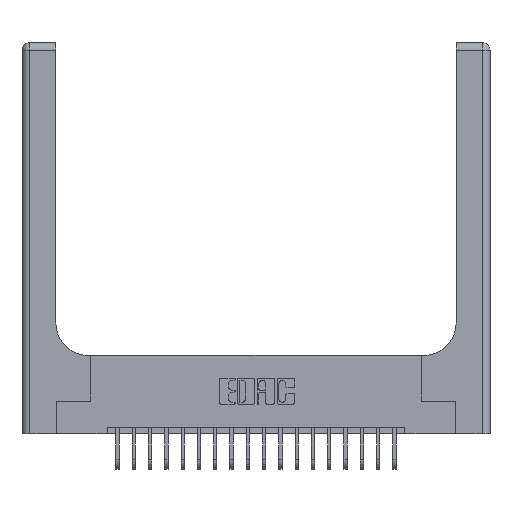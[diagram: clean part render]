
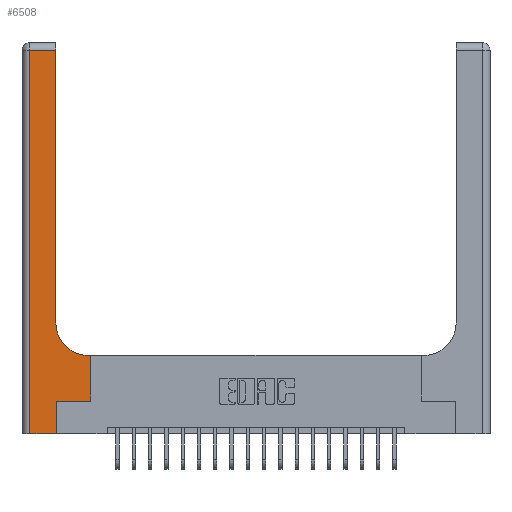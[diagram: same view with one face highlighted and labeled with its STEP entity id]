
A CAD part, top view. The second image highlights one B-rep face of the part: STEP entity #6508.
In plain terms, the highlighted planar face has unit normal (0, 0, 1).
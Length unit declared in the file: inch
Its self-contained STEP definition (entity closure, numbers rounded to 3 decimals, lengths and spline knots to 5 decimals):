
#472 = EDGE_CURVE ( 'NONE', #2801, #19625, #3547, .T. ) ;
#615 = CARTESIAN_POINT ( 'NONE',  ( 0.265, 0., 0.37 ) ) ;
#683 = PLANE ( 'NONE',  #11475 ) ;
#1580 = DIRECTION ( 'NONE',  ( 1., 0., 0. ) ) ;
#1695 = DIRECTION ( 'NONE',  ( 0., -1., 0. ) ) ;
#1717 = EDGE_CURVE ( 'NONE', #19625, #13800, #10769, .T. ) ;
#1804 = VECTOR ( 'NONE', #12880, 39.37008 ) ;
#1889 = CARTESIAN_POINT ( 'NONE',  ( 0.528, 0.25, 0.37 ) ) ;
#2115 = FACE_OUTER_BOUND ( 'NONE', #16311, .T. ) ;
#2153 = EDGE_CURVE ( 'NONE', #5515, #14715, #13797, .T. ) ;
#2319 = EDGE_CURVE ( 'NONE', #13633, #2801, #19051, .T. ) ;
#2414 = ORIENTED_EDGE ( 'NONE', *, *, #12610, .T. ) ;
#2652 = CARTESIAN_POINT ( 'NONE',  ( 0.51, 0.6, 0.37 ) ) ;
#2801 = VERTEX_POINT ( 'NONE', #17411 ) ;
#3007 = VERTEX_POINT ( 'NONE', #2652 ) ;
#3537 = EDGE_CURVE ( 'NONE', #10166, #3007, #11063, .T. ) ;
#3547 = LINE ( 'NONE', #15643, #15716 ) ;
#3594 = EDGE_CURVE ( 'NONE', #14715, #10166, #6774, .T. ) ;
#3761 = VECTOR ( 'NONE', #5128, 39.37008 ) ;
#4103 = VECTOR ( 'NONE', #11408, 39.37008 ) ;
#4941 = ORIENTED_EDGE ( 'NONE', *, *, #2153, .T. ) ;
#5128 = DIRECTION ( 'NONE',  ( -1., 0., 0. ) ) ;
#5199 = CIRCLE ( 'NONE', #8436, 0.25 ) ;
#5515 = VERTEX_POINT ( 'NONE', #12678 ) ;
#6261 = VECTOR ( 'NONE', #7864, 39.37008 ) ;
#6306 = DIRECTION ( 'NONE',  ( 1., 0., 0. ) ) ;
#6508 = ADVANCED_FACE ( 'NONE', ( #2115 ), #683, .F. ) ;
#6555 = VERTEX_POINT ( 'NONE', #8511 ) ;
#6585 = CARTESIAN_POINT ( 'NONE',  ( 0.528, 0.25, 0.37 ) ) ;
#6631 = LINE ( 'NONE', #12851, #6261 ) ;
#6774 = LINE ( 'NONE', #1889, #15116 ) ;
#7864 = DIRECTION ( 'NONE',  ( 0., 1., 0. ) ) ;
#8000 = CARTESIAN_POINT ( 'NONE',  ( 0.06, 0., 0.37 ) ) ;
#8436 = AXIS2_PLACEMENT_3D ( 'NONE', #11306, #12644, #6306 ) ;
#8511 = CARTESIAN_POINT ( 'NONE',  ( 0.26, 0.85, 0.37 ) ) ;
#9161 = EDGE_CURVE ( 'NONE', #13800, #5515, #18616, .T. ) ;
#9781 = ORIENTED_EDGE ( 'NONE', *, *, #472, .T. ) ;
#10166 = VERTEX_POINT ( 'NONE', #10931 ) ;
#10769 = LINE ( 'NONE', #16954, #17042 ) ;
#10931 = CARTESIAN_POINT ( 'NONE',  ( 0.528, 0.6, 0.37 ) ) ;
#11063 = LINE ( 'NONE', #18856, #1804 ) ;
#11306 = CARTESIAN_POINT ( 'NONE',  ( 0.51, 0.85, 0.37 ) ) ;
#11408 = DIRECTION ( 'NONE',  ( 0., 1., 0. ) ) ;
#11475 = AXIS2_PLACEMENT_3D ( 'NONE', #17960, #13020, #16248 ) ;
#11671 = CARTESIAN_POINT ( 'NONE',  ( 0.26, 2.94, 0.37 ) ) ;
#12589 = CARTESIAN_POINT ( 'NONE',  ( 0., 2.94, 0.37 ) ) ;
#12610 = EDGE_CURVE ( 'NONE', #6555, #13633, #6631, .T. ) ;
#12644 = DIRECTION ( 'NONE',  ( 0., 0., -1. ) ) ;
#12678 = CARTESIAN_POINT ( 'NONE',  ( 0.265, 0.25, 0.37 ) ) ;
#12851 = CARTESIAN_POINT ( 'NONE',  ( 0.26, 3., 0.37 ) ) ;
#12880 = DIRECTION ( 'NONE',  ( -1., 0., 0. ) ) ;
#12958 = EDGE_CURVE ( 'NONE', #3007, #6555, #5199, .T. ) ;
#13020 = DIRECTION ( 'NONE',  ( 0., 0., -1. ) ) ;
#13633 = VERTEX_POINT ( 'NONE', #11671 ) ;
#13797 = LINE ( 'NONE', #19872, #16083 ) ;
#13800 = VERTEX_POINT ( 'NONE', #19874 ) ;
#14033 = DIRECTION ( 'NONE',  ( 1., 0., 0. ) ) ;
#14189 = ORIENTED_EDGE ( 'NONE', *, *, #9161, .T. ) ;
#14715 = VERTEX_POINT ( 'NONE', #6585 ) ;
#15004 = ORIENTED_EDGE ( 'NONE', *, *, #3594, .T. ) ;
#15116 = VECTOR ( 'NONE', #19057, 39.37008 ) ;
#15643 = CARTESIAN_POINT ( 'NONE',  ( 0.06, 3., 0.37 ) ) ;
#15716 = VECTOR ( 'NONE', #1695, 39.37008 ) ;
#16083 = VECTOR ( 'NONE', #1580, 39.37008 ) ;
#16180 = ORIENTED_EDGE ( 'NONE', *, *, #3537, .T. ) ;
#16248 = DIRECTION ( 'NONE',  ( -1., 0., 0. ) ) ;
#16311 = EDGE_LOOP ( 'NONE', ( #2414, #17262, #9781, #16590, #14189, #4941, #15004, #16180, #17582 ) ) ;
#16590 = ORIENTED_EDGE ( 'NONE', *, *, #1717, .T. ) ;
#16954 = CARTESIAN_POINT ( 'NONE',  ( 0., 0., 0.37 ) ) ;
#17042 = VECTOR ( 'NONE', #14033, 39.37008 ) ;
#17262 = ORIENTED_EDGE ( 'NONE', *, *, #2319, .T. ) ;
#17411 = CARTESIAN_POINT ( 'NONE',  ( 0.06, 2.94, 0.37 ) ) ;
#17582 = ORIENTED_EDGE ( 'NONE', *, *, #12958, .T. ) ;
#17960 = CARTESIAN_POINT ( 'NONE',  ( 0., 3., 0.37 ) ) ;
#18616 = LINE ( 'NONE', #615, #4103 ) ;
#18856 = CARTESIAN_POINT ( 'NONE',  ( 0.26, 0.6, 0.37 ) ) ;
#19051 = LINE ( 'NONE', #12589, #3761 ) ;
#19057 = DIRECTION ( 'NONE',  ( 0., 1., 0. ) ) ;
#19625 = VERTEX_POINT ( 'NONE', #8000 ) ;
#19872 = CARTESIAN_POINT ( 'NONE',  ( 0.265, 0.25, 0.37 ) ) ;
#19874 = CARTESIAN_POINT ( 'NONE',  ( 0.265, 0., 0.37 ) ) ;
